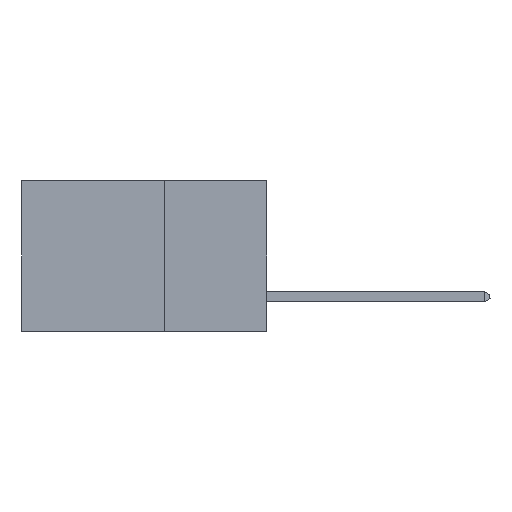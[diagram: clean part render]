
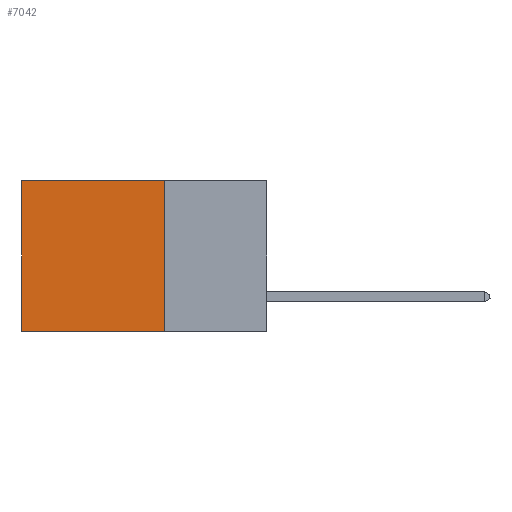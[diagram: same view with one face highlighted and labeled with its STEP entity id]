
A CAD part, left-side view. The second image highlights one B-rep face of the part: STEP entity #7042.
In plain terms, the highlighted planar face has unit normal (-1, 0, 0).
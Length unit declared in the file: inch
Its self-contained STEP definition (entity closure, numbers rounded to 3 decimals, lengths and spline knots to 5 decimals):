
#74 = VERTEX_POINT ( 'NONE', #11284 ) ;
#487 = VECTOR ( 'NONE', #17316, 39.37008 ) ;
#737 = DIRECTION ( 'NONE',  ( 0., 1., 0. ) ) ;
#1081 = EDGE_CURVE ( 'NONE', #27956, #12281, #14850, .T. ) ;
#1330 = LINE ( 'NONE', #31172, #487 ) ;
#1823 = DIRECTION ( 'NONE',  ( 0., 0., -1. ) ) ;
#3363 = ORIENTED_EDGE ( 'NONE', *, *, #1081, .F. ) ;
#4277 = DIRECTION ( 'NONE',  ( 1., 0., 0. ) ) ;
#5203 = LINE ( 'NONE', #18625, #33000 ) ;
#6090 = ORIENTED_EDGE ( 'NONE', *, *, #6438, .T. ) ;
#6438 = EDGE_CURVE ( 'NONE', #24279, #74, #5203, .T. ) ;
#7042 = ADVANCED_FACE ( 'NONE', ( #16035 ), #15601, .F. ) ;
#7357 = ORIENTED_EDGE ( 'NONE', *, *, #8011, .T. ) ;
#7753 = CARTESIAN_POINT ( 'NONE',  ( 0.2875, 0.25, 0. ) ) ;
#8011 = EDGE_CURVE ( 'NONE', #27956, #24279, #14657, .T. ) ;
#8105 = VECTOR ( 'NONE', #737, 39.37008 ) ;
#11284 = CARTESIAN_POINT ( 'NONE',  ( 0.2875, 0.6, -0.37 ) ) ;
#12146 = EDGE_LOOP ( 'NONE', ( #6090, #34177, #3363, #7357 ) ) ;
#12281 = VERTEX_POINT ( 'NONE', #15126 ) ;
#13042 = CARTESIAN_POINT ( 'NONE',  ( 0.2875, 0.25, 0. ) ) ;
#14657 = LINE ( 'NONE', #17312, #8105 ) ;
#14850 = LINE ( 'NONE', #20735, #35220 ) ;
#15126 = CARTESIAN_POINT ( 'NONE',  ( 0.2875, 0.25, -0.37 ) ) ;
#15541 = EDGE_CURVE ( 'NONE', #12281, #74, #1330, .T. ) ;
#15601 = PLANE ( 'NONE',  #18377 ) ;
#16035 = FACE_OUTER_BOUND ( 'NONE', #12146, .T. ) ;
#17312 = CARTESIAN_POINT ( 'NONE',  ( 0.2875, 0.25, 0. ) ) ;
#17316 = DIRECTION ( 'NONE',  ( 0., 1., 0. ) ) ;
#18377 = AXIS2_PLACEMENT_3D ( 'NONE', #13042, #4277, #18580 ) ;
#18580 = DIRECTION ( 'NONE',  ( 0., 0., -1. ) ) ;
#18625 = CARTESIAN_POINT ( 'NONE',  ( 0.2875, 0.6, 0. ) ) ;
#18987 = DIRECTION ( 'NONE',  ( 0., 0., -1. ) ) ;
#20735 = CARTESIAN_POINT ( 'NONE',  ( 0.2875, 0.25, 0. ) ) ;
#24279 = VERTEX_POINT ( 'NONE', #27636 ) ;
#27636 = CARTESIAN_POINT ( 'NONE',  ( 0.2875, 0.6, 0. ) ) ;
#27956 = VERTEX_POINT ( 'NONE', #7753 ) ;
#31172 = CARTESIAN_POINT ( 'NONE',  ( 0.2875, 0.25, -0.37 ) ) ;
#33000 = VECTOR ( 'NONE', #18987, 39.37008 ) ;
#34177 = ORIENTED_EDGE ( 'NONE', *, *, #15541, .F. ) ;
#35220 = VECTOR ( 'NONE', #1823, 39.37008 ) ;
